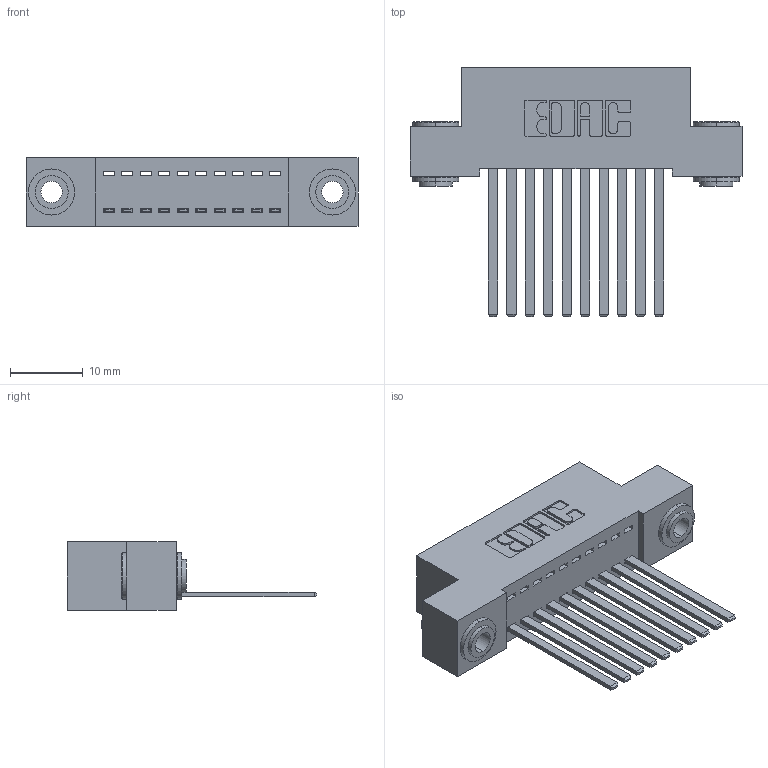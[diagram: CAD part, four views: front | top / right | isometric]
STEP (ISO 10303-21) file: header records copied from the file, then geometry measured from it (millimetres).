
FILE_DESCRIPTION (( 'STEP AP203' ), '1' );
FILE_NAME ('342-010-544-103.STEP', '2019-10-01T14:08:49', ( '' ), ( '' ), 'SwSTEP 2.0', 'SolidWorks 2016', '' );
FILE_SCHEMA (( 'CONFIG_CONTROL_DESIGN' ));
Length unit declared in the file: inch
Products named in the file (4): 345-292-001_345-293-144; 342-250-002_345-250-002-102; 342-010-544-103; 342 Part_.156 TH
Assembly tree (13 placements, depth 2):
  342-010-544-103
    342 Part_.156 TH
    345-292-001_345-293-144  x10
    342-250-002_345-250-002-102  x2
Bounding box: 45.72 x 34.3 x 9.4 mm (x, y, z)
Volume: 4029.5 mm3; surface area: 5875.4 mm2
Topology: 13 solids, 13 shells, 668 faces, 1955 edges, 1286 vertices
Faces by surface type: plane 456, cylinder 204, cone 8
Entity records: 10586 total; most frequent: CARTESIAN_POINT 1807, ORIENTED_EDGE 1746, DIRECTION 1619, EDGE_CURVE 873, LINE 725, VECTOR 725, VERTEX_POINT 578, AXIS2_PLACEMENT_3D 447
